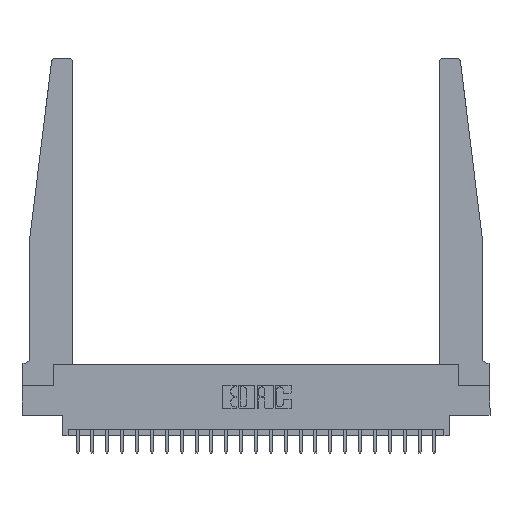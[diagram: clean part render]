
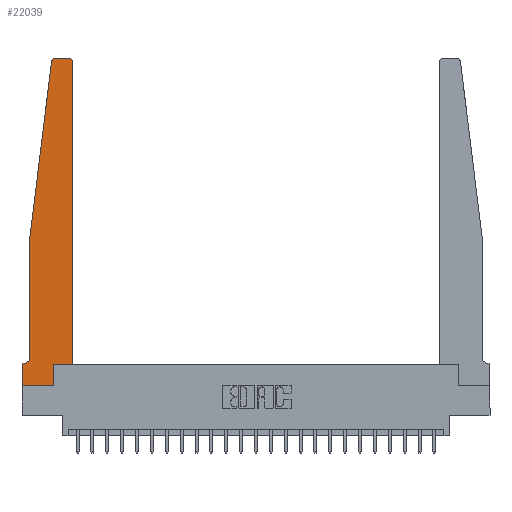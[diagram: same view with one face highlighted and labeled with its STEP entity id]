
A CAD part, top view. The second image highlights one B-rep face of the part: STEP entity #22039.
In plain terms, the highlighted planar face has unit normal (0, 0, 1).
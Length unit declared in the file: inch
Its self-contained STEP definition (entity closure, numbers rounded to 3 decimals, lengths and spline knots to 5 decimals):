
#236 = DIRECTION ( 'NONE',  ( 0., 0., 1. ) ) ;
#290 = EDGE_CURVE ( 'NONE', #22366, #1949, #20523, .T. ) ;
#345 = EDGE_CURVE ( 'NONE', #10467, #22366, #7529, .T. ) ;
#405 = EDGE_CURVE ( 'NONE', #13486, #7171, #10271, .T. ) ;
#414 = DIRECTION ( 'NONE',  ( 0., 0., 1. ) ) ;
#686 = CARTESIAN_POINT ( 'NONE',  ( 0.27653, 2.75, 0.37 ) ) ;
#1020 = VERTEX_POINT ( 'NONE', #10215 ) ;
#1407 = DIRECTION ( 'NONE',  ( -1., 0., 0. ) ) ;
#1600 = CARTESIAN_POINT ( 'NONE',  ( 0.425, 0.18, 0.37 ) ) ;
#1829 = ORIENTED_EDGE ( 'NONE', *, *, #20175, .T. ) ;
#1949 = VERTEX_POINT ( 'NONE', #10284 ) ;
#1971 = CARTESIAN_POINT ( 'NONE',  ( 0.015, 0.2375, 0.37 ) ) ;
#2145 = CARTESIAN_POINT ( 'NONE',  ( 0.065, 0.2375, 0.37 ) ) ;
#2181 = VECTOR ( 'NONE', #3018, 39.37008 ) ;
#2229 = DIRECTION ( 'NONE',  ( 1., 0., 0. ) ) ;
#2275 = DIRECTION ( 'NONE',  ( 1., 0., 0. ) ) ;
#2685 = VERTEX_POINT ( 'NONE', #1600 ) ;
#3018 = DIRECTION ( 'NONE',  ( 0., -1., 0. ) ) ;
#3112 = DIRECTION ( 'NONE',  ( 0., -1., 0. ) ) ;
#3162 = ORIENTED_EDGE ( 'NONE', *, *, #345, .T. ) ;
#3202 = EDGE_CURVE ( 'NONE', #4665, #13486, #9769, .T. ) ;
#3447 = FACE_OUTER_BOUND ( 'NONE', #9297, .T. ) ;
#3654 = CARTESIAN_POINT ( 'NONE',  ( 0.015, 0.1875, 0.37 ) ) ;
#3983 = VECTOR ( 'NONE', #9373, 39.37008 ) ;
#4174 = AXIS2_PLACEMENT_3D ( 'NONE', #1971, #11289, #13225 ) ;
#4360 = VERTEX_POINT ( 'NONE', #17262 ) ;
#4455 = VECTOR ( 'NONE', #21710, 39.37008 ) ;
#4555 = CIRCLE ( 'NONE', #4174, 0.05 ) ;
#4665 = VERTEX_POINT ( 'NONE', #16528 ) ;
#5306 = LINE ( 'NONE', #18318, #2181 ) ;
#5489 = CARTESIAN_POINT ( 'NONE',  ( 0.2605, 0., 0.37 ) ) ;
#5636 = EDGE_CURVE ( 'NONE', #2685, #14304, #6751, .T. ) ;
#5787 = CARTESIAN_POINT ( 'NONE',  ( 0., 0., 0.37 ) ) ;
#5964 = CARTESIAN_POINT ( 'NONE',  ( 0.395, 2.72, 0.37 ) ) ;
#6002 = ORIENTED_EDGE ( 'NONE', *, *, #21110, .T. ) ;
#6631 = DIRECTION ( 'NONE',  ( 0., 1., 0. ) ) ;
#6681 = EDGE_CURVE ( 'NONE', #1949, #8366, #5306, .T. ) ;
#6751 = LINE ( 'NONE', #17832, #4455 ) ;
#6797 = CARTESIAN_POINT ( 'NONE',  ( 0.24675, 2.72367, 0.37 ) ) ;
#6937 = AXIS2_PLACEMENT_3D ( 'NONE', #10833, #14240, #18384 ) ;
#7171 = VERTEX_POINT ( 'NONE', #19758 ) ;
#7178 = EDGE_CURVE ( 'NONE', #4360, #4665, #8801, .T. ) ;
#7529 = CIRCLE ( 'NONE', #15268, 0.03 ) ;
#7555 = ORIENTED_EDGE ( 'NONE', *, *, #405, .T. ) ;
#7590 = AXIS2_PLACEMENT_3D ( 'NONE', #5964, #414, #2229 ) ;
#7633 = DIRECTION ( 'NONE',  ( 1., 0., 0. ) ) ;
#7992 = VECTOR ( 'NONE', #3112, 39.37008 ) ;
#8053 = ORIENTED_EDGE ( 'NONE', *, *, #6681, .T. ) ;
#8095 = CARTESIAN_POINT ( 'NONE',  ( 0.2605, 0.18, 0.37 ) ) ;
#8341 = VECTOR ( 'NONE', #6631, 39.37008 ) ;
#8366 = VERTEX_POINT ( 'NONE', #2145 ) ;
#8801 = LINE ( 'NONE', #14385, #7992 ) ;
#9144 = LINE ( 'NONE', #10851, #3983 ) ;
#9297 = EDGE_LOOP ( 'NONE', ( #9803, #3162, #14906, #8053, #1829, #6002, #23057, #16301, #7555, #17144, #15835, #17030 ) ) ;
#9373 = DIRECTION ( 'NONE',  ( -1., 0., 0. ) ) ;
#9769 = LINE ( 'NONE', #5787, #20305 ) ;
#9803 = ORIENTED_EDGE ( 'NONE', *, *, #10634, .T. ) ;
#10215 = CARTESIAN_POINT ( 'NONE',  ( 0.395, 2.75, 0.37 ) ) ;
#10271 = LINE ( 'NONE', #8095, #8341 ) ;
#10284 = CARTESIAN_POINT ( 'NONE',  ( 0.065, 1.25, 0.37 ) ) ;
#10467 = VERTEX_POINT ( 'NONE', #686 ) ;
#10634 = EDGE_CURVE ( 'NONE', #1020, #10467, #9144, .T. ) ;
#10833 = CARTESIAN_POINT ( 'NONE',  ( 0., 0.1875, 0.37 ) ) ;
#10851 = CARTESIAN_POINT ( 'NONE',  ( 0.25, 2.75, 0.37 ) ) ;
#11289 = DIRECTION ( 'NONE',  ( 0., 0., -1. ) ) ;
#11371 = CARTESIAN_POINT ( 'NONE',  ( 0.065, 1.25, 0.37 ) ) ;
#11450 = CIRCLE ( 'NONE', #7590, 0.03 ) ;
#11554 = LINE ( 'NONE', #11662, #13774 ) ;
#11662 = CARTESIAN_POINT ( 'NONE',  ( 0.425, 0.18, 0.37 ) ) ;
#13225 = DIRECTION ( 'NONE',  ( -1., 0., 0. ) ) ;
#13486 = VERTEX_POINT ( 'NONE', #5489 ) ;
#13774 = VECTOR ( 'NONE', #17405, 39.37008 ) ;
#14240 = DIRECTION ( 'NONE',  ( 0., 0., 1. ) ) ;
#14304 = VERTEX_POINT ( 'NONE', #17731 ) ;
#14385 = CARTESIAN_POINT ( 'NONE',  ( 0., 0., 0.37 ) ) ;
#14906 = ORIENTED_EDGE ( 'NONE', *, *, #290, .T. ) ;
#15209 = VERTEX_POINT ( 'NONE', #3654 ) ;
#15268 = AXIS2_PLACEMENT_3D ( 'NONE', #16860, #236, #7633 ) ;
#15835 = ORIENTED_EDGE ( 'NONE', *, *, #5636, .T. ) ;
#16226 = LINE ( 'NONE', #19495, #18188 ) ;
#16301 = ORIENTED_EDGE ( 'NONE', *, *, #3202, .T. ) ;
#16429 = PLANE ( 'NONE',  #6937 ) ;
#16528 = CARTESIAN_POINT ( 'NONE',  ( 0., 0., 0.37 ) ) ;
#16558 = EDGE_CURVE ( 'NONE', #14304, #1020, #11450, .T. ) ;
#16574 = EDGE_CURVE ( 'NONE', #7171, #2685, #11554, .T. ) ;
#16860 = CARTESIAN_POINT ( 'NONE',  ( 0.27653, 2.72, 0.37 ) ) ;
#16984 = DIRECTION ( 'NONE',  ( -0.122, -0.992, 0. ) ) ;
#17030 = ORIENTED_EDGE ( 'NONE', *, *, #16558, .T. ) ;
#17144 = ORIENTED_EDGE ( 'NONE', *, *, #16574, .T. ) ;
#17262 = CARTESIAN_POINT ( 'NONE',  ( 0., 0.1875, 0.37 ) ) ;
#17405 = DIRECTION ( 'NONE',  ( 1., 0., 0. ) ) ;
#17731 = CARTESIAN_POINT ( 'NONE',  ( 0.425, 2.72, 0.37 ) ) ;
#17832 = CARTESIAN_POINT ( 'NONE',  ( 0.425, 0.18, 0.37 ) ) ;
#18188 = VECTOR ( 'NONE', #1407, 39.37008 ) ;
#18318 = CARTESIAN_POINT ( 'NONE',  ( 0.065, 1.25, 0.37 ) ) ;
#18384 = DIRECTION ( 'NONE',  ( 1., 0., 0. ) ) ;
#19163 = VECTOR ( 'NONE', #16984, 39.37008 ) ;
#19495 = CARTESIAN_POINT ( 'NONE',  ( 0.065, 0.1875, 0.37 ) ) ;
#19758 = CARTESIAN_POINT ( 'NONE',  ( 0.2605, 0.18, 0.37 ) ) ;
#20175 = EDGE_CURVE ( 'NONE', #8366, #15209, #4555, .T. ) ;
#20305 = VECTOR ( 'NONE', #2275, 39.37008 ) ;
#20523 = LINE ( 'NONE', #11371, #19163 ) ;
#21110 = EDGE_CURVE ( 'NONE', #15209, #4360, #16226, .T. ) ;
#21710 = DIRECTION ( 'NONE',  ( 0., 1., 0. ) ) ;
#22039 = ADVANCED_FACE ( 'NONE', ( #3447 ), #16429, .T. ) ;
#22366 = VERTEX_POINT ( 'NONE', #6797 ) ;
#23057 = ORIENTED_EDGE ( 'NONE', *, *, #7178, .T. ) ;
